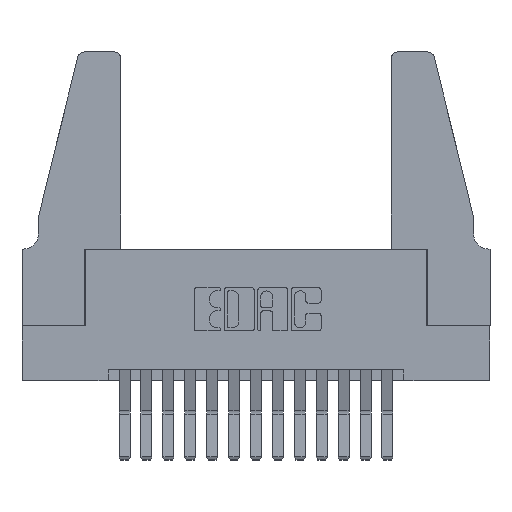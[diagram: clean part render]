
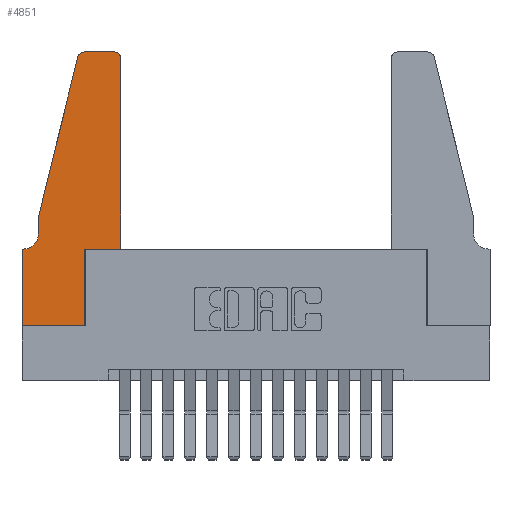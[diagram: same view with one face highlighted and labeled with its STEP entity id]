
A CAD part, top view. The second image highlights one B-rep face of the part: STEP entity #4851.
In plain terms, the highlighted planar face has unit normal (0, 0, 1).
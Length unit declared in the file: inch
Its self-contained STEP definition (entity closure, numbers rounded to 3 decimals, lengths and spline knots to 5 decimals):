
#66 = EDGE_CURVE ( 'NONE', #6632, #949, #11963, .T. ) ;
#326 = AXIS2_PLACEMENT_3D ( 'NONE', #10768, #3165, #12028 ) ;
#567 = CARTESIAN_POINT ( 'NONE',  ( 0.4205, 1.22, 0.37 ) ) ;
#643 = DIRECTION ( 'NONE',  ( 1., 0., 0. ) ) ;
#770 = ORIENTED_EDGE ( 'NONE', *, *, #3267, .T. ) ;
#898 = DIRECTION ( 'NONE',  ( 0., 0., 1. ) ) ;
#949 = VERTEX_POINT ( 'NONE', #13839 ) ;
#1130 = VERTEX_POINT ( 'NONE', #10891 ) ;
#1338 = DIRECTION ( 'NONE',  ( -1., 0., 0. ) ) ;
#1761 = VERTEX_POINT ( 'NONE', #10315 ) ;
#1803 = DIRECTION ( 'NONE',  ( 0., 0., 1. ) ) ;
#2112 = VERTEX_POINT ( 'NONE', #10785 ) ;
#2280 = AXIS2_PLACEMENT_3D ( 'NONE', #567, #1803, #643 ) ;
#2444 = LINE ( 'NONE', #12849, #15386 ) ;
#2471 = LINE ( 'NONE', #5726, #14670 ) ;
#2559 = CARTESIAN_POINT ( 'NONE',  ( 0.0755, 0.42, 0.37 ) ) ;
#2621 = ORIENTED_EDGE ( 'NONE', *, *, #13318, .T. ) ;
#2744 = ORIENTED_EDGE ( 'NONE', *, *, #13504, .T. ) ;
#3161 = VECTOR ( 'NONE', #9803, 39.37008 ) ;
#3165 = DIRECTION ( 'NONE',  ( 0., 0., -1. ) ) ;
#3267 = EDGE_CURVE ( 'NONE', #2112, #1130, #4294, .T. ) ;
#3732 = LINE ( 'NONE', #13133, #10069 ) ;
#4077 = EDGE_CURVE ( 'NONE', #15736, #8420, #2444, .T. ) ;
#4291 = ORIENTED_EDGE ( 'NONE', *, *, #14304, .T. ) ;
#4294 = CIRCLE ( 'NONE', #2280, 0.03 ) ;
#4321 = VECTOR ( 'NONE', #6784, 39.37008 ) ;
#4851 = ADVANCED_FACE ( 'NONE', ( #11167 ), #10514, .T. ) ;
#4946 = DIRECTION ( 'NONE',  ( -1., 0., 0. ) ) ;
#5276 = VECTOR ( 'NONE', #10211, 39.37008 ) ;
#5417 = CIRCLE ( 'NONE', #326, 0.07 ) ;
#5532 = CARTESIAN_POINT ( 'NONE',  ( 0.4505, 0.35, 0.37 ) ) ;
#5726 = CARTESIAN_POINT ( 'NONE',  ( 0.0755, 0.5, 0.37 ) ) ;
#5779 = DIRECTION ( 'NONE',  ( 0., -1., 0. ) ) ;
#5790 = ORIENTED_EDGE ( 'NONE', *, *, #10125, .T. ) ;
#5849 = LINE ( 'NONE', #6493, #6238 ) ;
#6073 = AXIS2_PLACEMENT_3D ( 'NONE', #6754, #15436, #8013 ) ;
#6238 = VECTOR ( 'NONE', #7760, 39.37008 ) ;
#6418 = ORIENTED_EDGE ( 'NONE', *, *, #8674, .T. ) ;
#6493 = CARTESIAN_POINT ( 'NONE',  ( 0.4505, 0.35, 0.37 ) ) ;
#6505 = CARTESIAN_POINT ( 'NONE',  ( 0.4505, 0.35, 0.37 ) ) ;
#6632 = VERTEX_POINT ( 'NONE', #7975 ) ;
#6754 = CARTESIAN_POINT ( 'NONE',  ( 0., 0.35, 0.37 ) ) ;
#6784 = DIRECTION ( 'NONE',  ( 1., 0., 0. ) ) ;
#6884 = EDGE_CURVE ( 'NONE', #1761, #6632, #14558, .T. ) ;
#7693 = LINE ( 'NONE', #15843, #13932 ) ;
#7760 = DIRECTION ( 'NONE',  ( 0., 1., 0. ) ) ;
#7786 = LINE ( 'NONE', #11218, #10363 ) ;
#7975 = CARTESIAN_POINT ( 'NONE',  ( 0.25487, 1.22718, 0.37 ) ) ;
#8013 = DIRECTION ( 'NONE',  ( 1., 0., 0. ) ) ;
#8063 = VERTEX_POINT ( 'NONE', #15741 ) ;
#8420 = VERTEX_POINT ( 'NONE', #9193 ) ;
#8579 = CARTESIAN_POINT ( 'NONE',  ( 0.284, 1.22, 0.37 ) ) ;
#8674 = EDGE_CURVE ( 'NONE', #12934, #10782, #7693, .T. ) ;
#9193 = CARTESIAN_POINT ( 'NONE',  ( 0., 0., 0.37 ) ) ;
#9554 = VERTEX_POINT ( 'NONE', #6505 ) ;
#9803 = DIRECTION ( 'NONE',  ( 1., 0., 0. ) ) ;
#9844 = DIRECTION ( 'NONE',  ( 1., 0., 0. ) ) ;
#9875 = CARTESIAN_POINT ( 'NONE',  ( 0.0755, 0.5, 0.37 ) ) ;
#9917 = LINE ( 'NONE', #11025, #3161 ) ;
#10069 = VECTOR ( 'NONE', #1338, 39.37008 ) ;
#10125 = EDGE_CURVE ( 'NONE', #9554, #2112, #5849, .T. ) ;
#10211 = DIRECTION ( 'NONE',  ( -0.239, -0.971, 0. ) ) ;
#10315 = CARTESIAN_POINT ( 'NONE',  ( 0.284, 1.25, 0.37 ) ) ;
#10363 = VECTOR ( 'NONE', #4946, 39.37008 ) ;
#10420 = DIRECTION ( 'NONE',  ( 0., -1., 0. ) ) ;
#10514 = PLANE ( 'NONE',  #6073 ) ;
#10709 = VERTEX_POINT ( 'NONE', #2559 ) ;
#10768 = CARTESIAN_POINT ( 'NONE',  ( 0.0055, 0.42, 0.37 ) ) ;
#10782 = VERTEX_POINT ( 'NONE', #14001 ) ;
#10785 = CARTESIAN_POINT ( 'NONE',  ( 0.4505, 1.22, 0.37 ) ) ;
#10891 = CARTESIAN_POINT ( 'NONE',  ( 0.4205, 1.25, 0.37 ) ) ;
#10960 = DIRECTION ( 'NONE',  ( 0., 1., 0. ) ) ;
#11020 = EDGE_CURVE ( 'NONE', #10709, #8063, #5417, .T. ) ;
#11025 = CARTESIAN_POINT ( 'NONE',  ( 0., 0., 0.37 ) ) ;
#11167 = FACE_OUTER_BOUND ( 'NONE', #15039, .T. ) ;
#11218 = CARTESIAN_POINT ( 'NONE',  ( 0.0755, 0.35, 0.37 ) ) ;
#11538 = CARTESIAN_POINT ( 'NONE',  ( 0., 0.35, 0.37 ) ) ;
#11827 = EDGE_CURVE ( 'NONE', #8420, #12934, #9917, .T. ) ;
#11963 = LINE ( 'NONE', #9875, #5276 ) ;
#11998 = ORIENTED_EDGE ( 'NONE', *, *, #6884, .T. ) ;
#12028 = DIRECTION ( 'NONE',  ( -1., 0., 0. ) ) ;
#12831 = ORIENTED_EDGE ( 'NONE', *, *, #11827, .T. ) ;
#12849 = CARTESIAN_POINT ( 'NONE',  ( 0., 0., 0.37 ) ) ;
#12934 = VERTEX_POINT ( 'NONE', #15650 ) ;
#13133 = CARTESIAN_POINT ( 'NONE',  ( 0.2605, 1.25, 0.37 ) ) ;
#13318 = EDGE_CURVE ( 'NONE', #1130, #1761, #3732, .T. ) ;
#13504 = EDGE_CURVE ( 'NONE', #10782, #9554, #13919, .T. ) ;
#13839 = CARTESIAN_POINT ( 'NONE',  ( 0.0755, 0.5, 0.37 ) ) ;
#13919 = LINE ( 'NONE', #5532, #4321 ) ;
#13932 = VECTOR ( 'NONE', #10960, 39.37008 ) ;
#14001 = CARTESIAN_POINT ( 'NONE',  ( 0.2865, 0.35, 0.37 ) ) ;
#14101 = ORIENTED_EDGE ( 'NONE', *, *, #4077, .T. ) ;
#14304 = EDGE_CURVE ( 'NONE', #949, #10709, #2471, .T. ) ;
#14558 = CIRCLE ( 'NONE', #15881, 0.03 ) ;
#14670 = VECTOR ( 'NONE', #5779, 39.37008 ) ;
#14884 = ORIENTED_EDGE ( 'NONE', *, *, #15534, .T. ) ;
#15039 = EDGE_LOOP ( 'NONE', ( #2621, #11998, #16348, #4291, #15085, #14884, #14101, #12831, #6418, #2744, #5790, #770 ) ) ;
#15085 = ORIENTED_EDGE ( 'NONE', *, *, #11020, .T. ) ;
#15386 = VECTOR ( 'NONE', #10420, 39.37008 ) ;
#15436 = DIRECTION ( 'NONE',  ( 0., 0., 1. ) ) ;
#15534 = EDGE_CURVE ( 'NONE', #8063, #15736, #7786, .T. ) ;
#15650 = CARTESIAN_POINT ( 'NONE',  ( 0.2865, 0., 0.37 ) ) ;
#15736 = VERTEX_POINT ( 'NONE', #11538 ) ;
#15741 = CARTESIAN_POINT ( 'NONE',  ( 0.0055, 0.35, 0.37 ) ) ;
#15843 = CARTESIAN_POINT ( 'NONE',  ( 0.2865, 0.35, 0.37 ) ) ;
#15881 = AXIS2_PLACEMENT_3D ( 'NONE', #8579, #898, #9844 ) ;
#16348 = ORIENTED_EDGE ( 'NONE', *, *, #66, .T. ) ;
